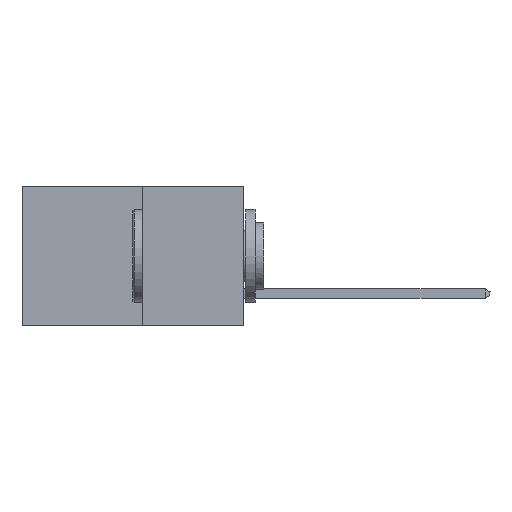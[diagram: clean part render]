
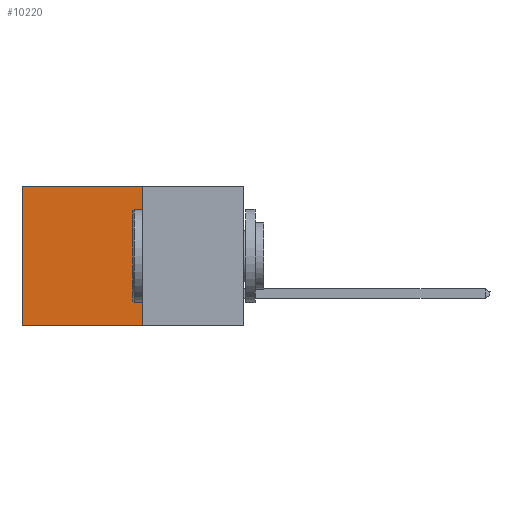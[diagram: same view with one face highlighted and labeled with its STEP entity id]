
A CAD part, left-side view. The second image highlights one B-rep face of the part: STEP entity #10220.
In plain terms, the highlighted planar face has unit normal (-1, 0, 0).
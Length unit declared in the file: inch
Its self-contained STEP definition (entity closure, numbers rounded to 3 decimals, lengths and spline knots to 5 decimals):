
#606 = ORIENTED_EDGE ( 'NONE', *, *, #2585, .T. ) ;
#761 = FACE_OUTER_BOUND ( 'NONE', #6275, .T. ) ;
#1118 = CARTESIAN_POINT ( 'NONE',  ( 0.277, 0.27, -0.37 ) ) ;
#1988 = VECTOR ( 'NONE', #20884, 39.37008 ) ;
#2526 = LINE ( 'NONE', #13174, #1988 ) ;
#2585 = EDGE_CURVE ( 'NONE', #16388, #15962, #17919, .T. ) ;
#2820 = DIRECTION ( 'NONE',  ( 1., 0., 0. ) ) ;
#3352 = CARTESIAN_POINT ( 'NONE',  ( 0.277, 0.27, -0.37 ) ) ;
#4708 = ORIENTED_EDGE ( 'NONE', *, *, #12744, .T. ) ;
#5114 = VECTOR ( 'NONE', #5356, 39.37008 ) ;
#5322 = EDGE_CURVE ( 'NONE', #9814, #19226, #5523, .T. ) ;
#5356 = DIRECTION ( 'NONE',  ( 0., 1., 0. ) ) ;
#5523 = LINE ( 'NONE', #17788, #13211 ) ;
#6118 = VECTOR ( 'NONE', #10844, 39.37008 ) ;
#6275 = EDGE_LOOP ( 'NONE', ( #4708, #9633, #18471, #606 ) ) ;
#6868 = CARTESIAN_POINT ( 'NONE',  ( 0.277, 0.59, 0. ) ) ;
#6923 = CARTESIAN_POINT ( 'NONE',  ( 0.277, 0.27, 0. ) ) ;
#9633 = ORIENTED_EDGE ( 'NONE', *, *, #5322, .F. ) ;
#9814 = VERTEX_POINT ( 'NONE', #3352 ) ;
#9952 = LINE ( 'NONE', #20210, #6118 ) ;
#10220 = ADVANCED_FACE ( 'NONE', ( #761 ), #11067, .F. ) ;
#10844 = DIRECTION ( 'NONE',  ( 0., 0., -1. ) ) ;
#11067 = PLANE ( 'NONE',  #17949 ) ;
#12744 = EDGE_CURVE ( 'NONE', #15962, #19226, #2526, .T. ) ;
#13174 = CARTESIAN_POINT ( 'NONE',  ( 0.277, 0.59, -0.37 ) ) ;
#13211 = VECTOR ( 'NONE', #20895, 39.37008 ) ;
#14328 = DIRECTION ( 'NONE',  ( 0., 0., -1. ) ) ;
#14735 = CARTESIAN_POINT ( 'NONE',  ( 0.277, 0.27, 0. ) ) ;
#15962 = VERTEX_POINT ( 'NONE', #6868 ) ;
#16388 = VERTEX_POINT ( 'NONE', #14735 ) ;
#16705 = CARTESIAN_POINT ( 'NONE',  ( 0.277, 0.59, -0.37 ) ) ;
#16729 = EDGE_CURVE ( 'NONE', #16388, #9814, #9952, .T. ) ;
#17788 = CARTESIAN_POINT ( 'NONE',  ( 0.277, 0.27, -0.37 ) ) ;
#17919 = LINE ( 'NONE', #6923, #5114 ) ;
#17949 = AXIS2_PLACEMENT_3D ( 'NONE', #1118, #2820, #14328 ) ;
#18471 = ORIENTED_EDGE ( 'NONE', *, *, #16729, .F. ) ;
#19226 = VERTEX_POINT ( 'NONE', #16705 ) ;
#20210 = CARTESIAN_POINT ( 'NONE',  ( 0.277, 0.27, -0.37 ) ) ;
#20884 = DIRECTION ( 'NONE',  ( 0., 0., -1. ) ) ;
#20895 = DIRECTION ( 'NONE',  ( 0., 1., 0. ) ) ;
